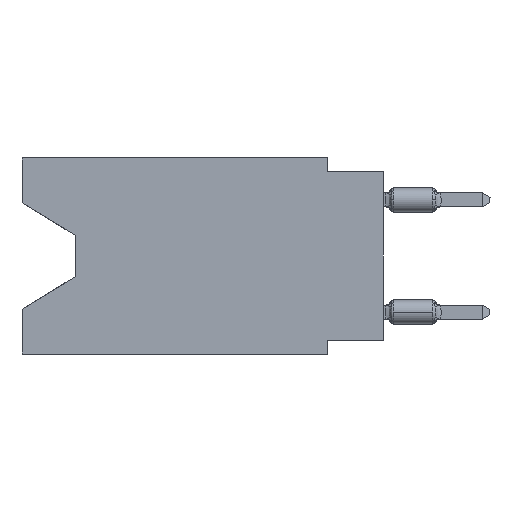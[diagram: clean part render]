
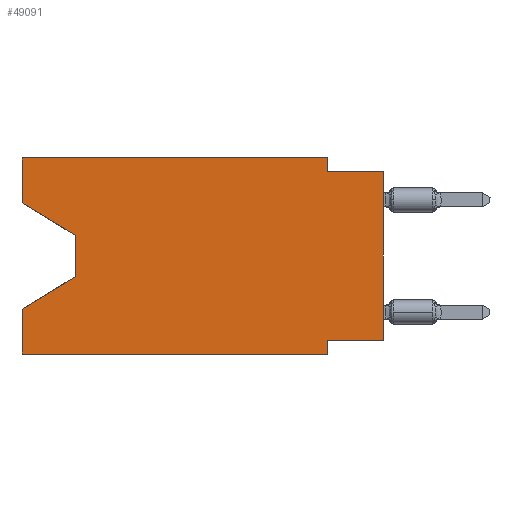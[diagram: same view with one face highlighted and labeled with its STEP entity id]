
A CAD part, left-side view. The second image highlights one B-rep face of the part: STEP entity #49091.
In plain terms, the highlighted planar face has unit normal (-1, 0, 0).
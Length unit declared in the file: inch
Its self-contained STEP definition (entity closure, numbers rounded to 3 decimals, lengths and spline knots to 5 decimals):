
#336 = DIRECTION ( 'NONE',  ( 0., 0., 1. ) ) ;
#708 = CARTESIAN_POINT ( 'NONE',  ( 0., 0.1, -0.35 ) ) ;
#1616 = VECTOR ( 'NONE', #25884, 39.37008 ) ;
#2580 = LINE ( 'NONE', #18178, #40964 ) ;
#5368 = CARTESIAN_POINT ( 'NONE',  ( 0., 0.1, 0. ) ) ;
#5408 = ORIENTED_EDGE ( 'NONE', *, *, #36633, .F. ) ;
#5548 = LINE ( 'NONE', #5880, #47274 ) ;
#5880 = CARTESIAN_POINT ( 'NONE',  ( 0., 0.645, 0. ) ) ;
#6063 = CARTESIAN_POINT ( 'NONE',  ( 0., 0.55, -0.212 ) ) ;
#6309 = EDGE_CURVE ( 'NONE', #53148, #26367, #52649, .T. ) ;
#6685 = DIRECTION ( 'NONE',  ( 1., 0., 0. ) ) ;
#7474 = DIRECTION ( 'NONE',  ( 0., 0., -1. ) ) ;
#7713 = VECTOR ( 'NONE', #58030, 39.37008 ) ;
#8434 = VERTEX_POINT ( 'NONE', #11073 ) ;
#8763 = EDGE_CURVE ( 'NONE', #44560, #27478, #40225, .T. ) ;
#9637 = LINE ( 'NONE', #29440, #7713 ) ;
#10720 = VECTOR ( 'NONE', #26254, 39.37008 ) ;
#11073 = CARTESIAN_POINT ( 'NONE',  ( 0., 0.645, -0.35 ) ) ;
#11130 = LINE ( 'NONE', #49452, #39401 ) ;
#11656 = DIRECTION ( 'NONE',  ( 0., -1., 0. ) ) ;
#11832 = LINE ( 'NONE', #5368, #33041 ) ;
#12735 = CARTESIAN_POINT ( 'NONE',  ( 0., 0., -0.325 ) ) ;
#13065 = VERTEX_POINT ( 'NONE', #54440 ) ;
#13112 = CARTESIAN_POINT ( 'NONE',  ( 0., 0.645, -0.35 ) ) ;
#14861 = EDGE_CURVE ( 'NONE', #55510, #44560, #5548, .T. ) ;
#14990 = EDGE_CURVE ( 'NONE', #49026, #13065, #17120, .T. ) ;
#15023 = EDGE_CURVE ( 'NONE', #8434, #57757, #24379, .T. ) ;
#15481 = EDGE_CURVE ( 'NONE', #55510, #42452, #49370, .T. ) ;
#15681 = DIRECTION ( 'NONE',  ( 0., 1., 0. ) ) ;
#16840 = CARTESIAN_POINT ( 'NONE',  ( 0., 0., -0.025 ) ) ;
#17120 = LINE ( 'NONE', #47622, #34866 ) ;
#18075 = EDGE_CURVE ( 'NONE', #27478, #38240, #11832, .T. ) ;
#18178 = CARTESIAN_POINT ( 'NONE',  ( 0., 0.1, -0.35 ) ) ;
#20072 = CARTESIAN_POINT ( 'NONE',  ( 0., 0.645, 0. ) ) ;
#20554 = ORIENTED_EDGE ( 'NONE', *, *, #14861, .F. ) ;
#21332 = ORIENTED_EDGE ( 'NONE', *, *, #43605, .F. ) ;
#21723 = LINE ( 'NONE', #16840, #53569 ) ;
#23471 = VECTOR ( 'NONE', #62455, 39.37008 ) ;
#24270 = EDGE_CURVE ( 'NONE', #42452, #49026, #54458, .T. ) ;
#24379 = LINE ( 'NONE', #13112, #23471 ) ;
#25884 = DIRECTION ( 'NONE',  ( 0., 0., -1. ) ) ;
#26037 = CARTESIAN_POINT ( 'NONE',  ( 0., 0.55, -0.138 ) ) ;
#26254 = DIRECTION ( 'NONE',  ( 0., -1., 0. ) ) ;
#26367 = VERTEX_POINT ( 'NONE', #61142 ) ;
#27120 = PLANE ( 'NONE',  #48683 ) ;
#27478 = VERTEX_POINT ( 'NONE', #48782 ) ;
#28983 = ORIENTED_EDGE ( 'NONE', *, *, #15023, .T. ) ;
#29440 = CARTESIAN_POINT ( 'NONE',  ( 0., 0.645, 0. ) ) ;
#29790 = CARTESIAN_POINT ( 'NONE',  ( 0., 0.55, -0.138 ) ) ;
#30252 = EDGE_LOOP ( 'NONE', ( #59909, #56083, #53331, #47329, #28983, #59612, #5408, #34292, #21332, #47138, #31596, #20554 ) ) ;
#30553 = CARTESIAN_POINT ( 'NONE',  ( 0., 0.1, -0.025 ) ) ;
#31360 = DIRECTION ( 'NONE',  ( 0., 0., -1. ) ) ;
#31596 = ORIENTED_EDGE ( 'NONE', *, *, #8763, .F. ) ;
#31666 = FACE_OUTER_BOUND ( 'NONE', #30252, .T. ) ;
#32260 = DIRECTION ( 'NONE',  ( 0., 0., -1. ) ) ;
#33041 = VECTOR ( 'NONE', #32260, 39.37008 ) ;
#34292 = ORIENTED_EDGE ( 'NONE', *, *, #6309, .T. ) ;
#34313 = CARTESIAN_POINT ( 'NONE',  ( 0., 0.645, -0.08025 ) ) ;
#34866 = VECTOR ( 'NONE', #57050, 39.37008 ) ;
#36633 = EDGE_CURVE ( 'NONE', #53148, #36948, #11130, .T. ) ;
#36948 = VERTEX_POINT ( 'NONE', #50591 ) ;
#38240 = VERTEX_POINT ( 'NONE', #30553 ) ;
#38404 = CARTESIAN_POINT ( 'NONE',  ( 0., 0.645, 0. ) ) ;
#39401 = VECTOR ( 'NONE', #15681, 39.37008 ) ;
#40225 = LINE ( 'NONE', #20072, #10720 ) ;
#40964 = VECTOR ( 'NONE', #7474, 39.37008 ) ;
#41945 = CARTESIAN_POINT ( 'NONE',  ( 0., 0., 0. ) ) ;
#42452 = VERTEX_POINT ( 'NONE', #26037 ) ;
#43605 = EDGE_CURVE ( 'NONE', #38240, #26367, #21723, .T. ) ;
#44560 = VERTEX_POINT ( 'NONE', #38404 ) ;
#45307 = VECTOR ( 'NONE', #60075, 39.37008 ) ;
#47138 = ORIENTED_EDGE ( 'NONE', *, *, #18075, .F. ) ;
#47274 = VECTOR ( 'NONE', #336, 39.37008 ) ;
#47329 = ORIENTED_EDGE ( 'NONE', *, *, #55631, .F. ) ;
#47558 = CARTESIAN_POINT ( 'NONE',  ( 0., 0.645, 0. ) ) ;
#47622 = CARTESIAN_POINT ( 'NONE',  ( 0., 0.55, -0.212 ) ) ;
#48683 = AXIS2_PLACEMENT_3D ( 'NONE', #47558, #6685, #31360 ) ;
#48782 = CARTESIAN_POINT ( 'NONE',  ( 0., 0.1, 0. ) ) ;
#49026 = VERTEX_POINT ( 'NONE', #6063 ) ;
#49091 = ADVANCED_FACE ( 'NONE', ( #31666 ), #27120, .F. ) ;
#49370 = LINE ( 'NONE', #49703, #45307 ) ;
#49452 = CARTESIAN_POINT ( 'NONE',  ( 0., 0., -0.325 ) ) ;
#49703 = CARTESIAN_POINT ( 'NONE',  ( 0., 0.645, -0.08025 ) ) ;
#50591 = CARTESIAN_POINT ( 'NONE',  ( 0., 0.1, -0.325 ) ) ;
#51099 = VECTOR ( 'NONE', #61752, 39.37008 ) ;
#52649 = LINE ( 'NONE', #41945, #51099 ) ;
#53148 = VERTEX_POINT ( 'NONE', #12735 ) ;
#53331 = ORIENTED_EDGE ( 'NONE', *, *, #14990, .T. ) ;
#53569 = VECTOR ( 'NONE', #11656, 39.37008 ) ;
#54440 = CARTESIAN_POINT ( 'NONE',  ( 0., 0.645, -0.26975 ) ) ;
#54458 = LINE ( 'NONE', #29790, #1616 ) ;
#55510 = VERTEX_POINT ( 'NONE', #34313 ) ;
#55631 = EDGE_CURVE ( 'NONE', #8434, #13065, #9637, .T. ) ;
#56083 = ORIENTED_EDGE ( 'NONE', *, *, #24270, .T. ) ;
#56218 = EDGE_CURVE ( 'NONE', #36948, #57757, #2580, .T. ) ;
#57050 = DIRECTION ( 'NONE',  ( 0., 0.855, -0.519 ) ) ;
#57757 = VERTEX_POINT ( 'NONE', #708 ) ;
#58030 = DIRECTION ( 'NONE',  ( 0., 0., 1. ) ) ;
#59612 = ORIENTED_EDGE ( 'NONE', *, *, #56218, .F. ) ;
#59909 = ORIENTED_EDGE ( 'NONE', *, *, #15481, .T. ) ;
#60075 = DIRECTION ( 'NONE',  ( 0., -0.855, -0.519 ) ) ;
#61142 = CARTESIAN_POINT ( 'NONE',  ( 0., 0., -0.025 ) ) ;
#61752 = DIRECTION ( 'NONE',  ( 0., 0., 1. ) ) ;
#62455 = DIRECTION ( 'NONE',  ( 0., -1., 0. ) ) ;
